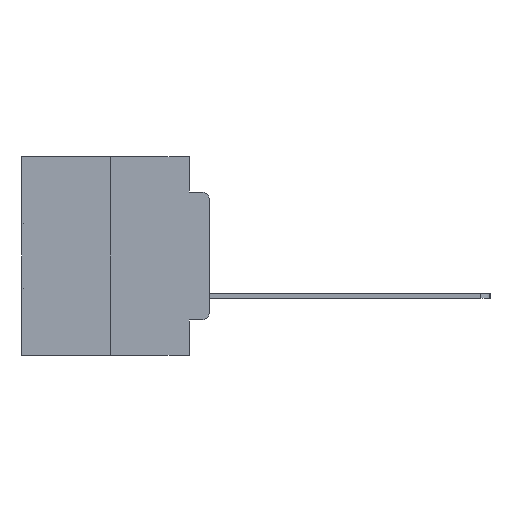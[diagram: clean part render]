
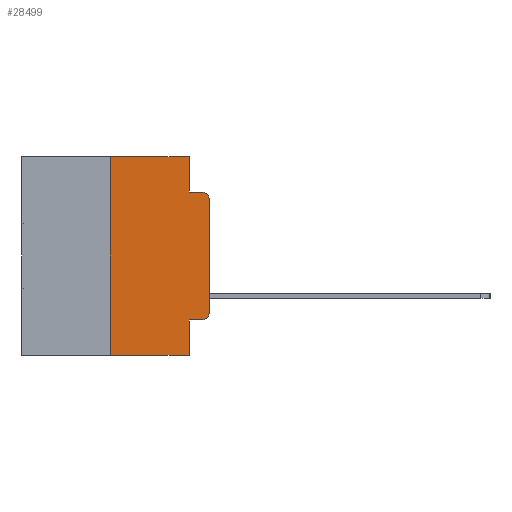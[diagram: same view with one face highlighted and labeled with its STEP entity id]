
A CAD part, left-side view. The second image highlights one B-rep face of the part: STEP entity #28499.
In plain terms, the highlighted planar face has unit normal (-1, 0, 0).
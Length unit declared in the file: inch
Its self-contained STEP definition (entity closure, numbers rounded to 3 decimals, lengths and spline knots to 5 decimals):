
#213 = CARTESIAN_POINT ( 'NONE',  ( 0., 0.02, -0.1085 ) ) ;
#919 = ORIENTED_EDGE ( 'NONE', *, *, #4600, .F. ) ;
#1004 = EDGE_LOOP ( 'NONE', ( #18325, #6069, #16161, #3114, #25255, #919, #17935, #4923, #3471, #26992 ) ) ;
#1137 = EDGE_CURVE ( 'NONE', #25202, #6873, #22551, .T. ) ;
#1201 = VERTEX_POINT ( 'NONE', #24159 ) ;
#1236 = CARTESIAN_POINT ( 'NONE',  ( 0., 0.051, 0. ) ) ;
#1256 = AXIS2_PLACEMENT_3D ( 'NONE', #26044, #12559, #28263 ) ;
#1947 = EDGE_CURVE ( 'NONE', #4671, #1201, #26779, .T. ) ;
#2197 = CARTESIAN_POINT ( 'NONE',  ( 0., 0.473, -0.5 ) ) ;
#2597 = DIRECTION ( 'NONE',  ( 0., 0., -1. ) ) ;
#3114 = ORIENTED_EDGE ( 'NONE', *, *, #23697, .F. ) ;
#3237 = VERTEX_POINT ( 'NONE', #17011 ) ;
#3417 = DIRECTION ( 'NONE',  ( 0., -1., 0. ) ) ;
#3471 = ORIENTED_EDGE ( 'NONE', *, *, #26192, .T. ) ;
#3637 = CARTESIAN_POINT ( 'NONE',  ( 0., 0.051, 0. ) ) ;
#4600 = EDGE_CURVE ( 'NONE', #4671, #25202, #4941, .T. ) ;
#4671 = VERTEX_POINT ( 'NONE', #14330 ) ;
#4902 = CARTESIAN_POINT ( 'NONE',  ( 0., 0.051, -0.4115 ) ) ;
#4923 = ORIENTED_EDGE ( 'NONE', *, *, #5903, .F. ) ;
#4941 = LINE ( 'NONE', #10071, #10447 ) ;
#5130 = CARTESIAN_POINT ( 'NONE',  ( 0., 0.02, -0.4115 ) ) ;
#5691 = AXIS2_PLACEMENT_3D ( 'NONE', #213, #16438, #2597 ) ;
#5903 = EDGE_CURVE ( 'NONE', #13832, #1201, #22442, .T. ) ;
#6069 = ORIENTED_EDGE ( 'NONE', *, *, #29288, .T. ) ;
#6700 = DIRECTION ( 'NONE',  ( 0., 0., 1. ) ) ;
#6873 = VERTEX_POINT ( 'NONE', #3637 ) ;
#7028 = DIRECTION ( 'NONE',  ( 0., 0., -1. ) ) ;
#8142 = DIRECTION ( 'NONE',  ( 0., 0., -1. ) ) ;
#9279 = DIRECTION ( 'NONE',  ( 0., -1., 0. ) ) ;
#9761 = VECTOR ( 'NONE', #13877, 39.37008 ) ;
#10071 = CARTESIAN_POINT ( 'NONE',  ( 0., 0.25, 0. ) ) ;
#10271 = CARTESIAN_POINT ( 'NONE',  ( 0., 0.25, 0. ) ) ;
#10447 = VECTOR ( 'NONE', #6700, 39.37008 ) ;
#10914 = CARTESIAN_POINT ( 'NONE',  ( 0., 0.051, -0.4115 ) ) ;
#11629 = CARTESIAN_POINT ( 'NONE',  ( 0., 0.473, 0. ) ) ;
#11756 = CARTESIAN_POINT ( 'NONE',  ( 0., 0.051, 0. ) ) ;
#12559 = DIRECTION ( 'NONE',  ( -1., 0., 0. ) ) ;
#13060 = FACE_OUTER_BOUND ( 'NONE', #1004, .T. ) ;
#13832 = VERTEX_POINT ( 'NONE', #10914 ) ;
#13877 = DIRECTION ( 'NONE',  ( 0., 0., 1. ) ) ;
#14184 = VERTEX_POINT ( 'NONE', #19039 ) ;
#14330 = CARTESIAN_POINT ( 'NONE',  ( 0., 0.25, -0.5 ) ) ;
#14562 = VERTEX_POINT ( 'NONE', #24772 ) ;
#14836 = CARTESIAN_POINT ( 'NONE',  ( 0., 0.02, -0.0885 ) ) ;
#15877 = LINE ( 'NONE', #27285, #9761 ) ;
#16003 = EDGE_CURVE ( 'NONE', #25725, #3237, #29301, .T. ) ;
#16050 = LINE ( 'NONE', #19537, #21341 ) ;
#16052 = EDGE_CURVE ( 'NONE', #14184, #16690, #16050, .T. ) ;
#16161 = ORIENTED_EDGE ( 'NONE', *, *, #16052, .F. ) ;
#16219 = DIRECTION ( 'NONE',  ( 0., 0., -1. ) ) ;
#16438 = DIRECTION ( 'NONE',  ( -1., 0., 0. ) ) ;
#16690 = VERTEX_POINT ( 'NONE', #14836 ) ;
#17011 = CARTESIAN_POINT ( 'NONE',  ( 0., 0., -0.3915 ) ) ;
#17935 = ORIENTED_EDGE ( 'NONE', *, *, #1947, .T. ) ;
#18325 = ORIENTED_EDGE ( 'NONE', *, *, #27883, .T. ) ;
#18706 = DIRECTION ( 'NONE',  ( 0., -1., 0. ) ) ;
#19039 = CARTESIAN_POINT ( 'NONE',  ( 0., 0.051, -0.0885 ) ) ;
#19145 = VECTOR ( 'NONE', #8142, 39.37008 ) ;
#19537 = CARTESIAN_POINT ( 'NONE',  ( 0., 0.051, -0.0885 ) ) ;
#19883 = LINE ( 'NONE', #1236, #19145 ) ;
#20569 = DIRECTION ( 'NONE',  ( 0., -1., 0. ) ) ;
#20880 = VECTOR ( 'NONE', #20569, 39.37008 ) ;
#21341 = VECTOR ( 'NONE', #3417, 39.37008 ) ;
#21862 = VECTOR ( 'NONE', #9279, 39.37008 ) ;
#22442 = LINE ( 'NONE', #11756, #27602 ) ;
#22551 = LINE ( 'NONE', #22916, #21862 ) ;
#22916 = CARTESIAN_POINT ( 'NONE',  ( 0., 0.473, 0. ) ) ;
#23376 = LINE ( 'NONE', #4902, #29241 ) ;
#23697 = EDGE_CURVE ( 'NONE', #6873, #14184, #19883, .T. ) ;
#24159 = CARTESIAN_POINT ( 'NONE',  ( 0., 0.051, -0.5 ) ) ;
#24772 = CARTESIAN_POINT ( 'NONE',  ( 0., 0., -0.1085 ) ) ;
#25202 = VERTEX_POINT ( 'NONE', #10271 ) ;
#25255 = ORIENTED_EDGE ( 'NONE', *, *, #1137, .F. ) ;
#25725 = VERTEX_POINT ( 'NONE', #5130 ) ;
#26044 = CARTESIAN_POINT ( 'NONE',  ( 0., 0.02, -0.3915 ) ) ;
#26192 = EDGE_CURVE ( 'NONE', #13832, #25725, #23376, .T. ) ;
#26779 = LINE ( 'NONE', #2197, #20880 ) ;
#26992 = ORIENTED_EDGE ( 'NONE', *, *, #16003, .T. ) ;
#27060 = CIRCLE ( 'NONE', #5691, 0.02 ) ;
#27285 = CARTESIAN_POINT ( 'NONE',  ( 0., 0., 0. ) ) ;
#27347 = PLANE ( 'NONE',  #27724 ) ;
#27602 = VECTOR ( 'NONE', #7028, 39.37008 ) ;
#27724 = AXIS2_PLACEMENT_3D ( 'NONE', #11629, #28920, #16219 ) ;
#27883 = EDGE_CURVE ( 'NONE', #3237, #14562, #15877, .T. ) ;
#28263 = DIRECTION ( 'NONE',  ( 0., 0., -1. ) ) ;
#28499 = ADVANCED_FACE ( 'NONE', ( #13060 ), #27347, .F. ) ;
#28920 = DIRECTION ( 'NONE',  ( 1., 0., 0. ) ) ;
#29241 = VECTOR ( 'NONE', #18706, 39.37008 ) ;
#29288 = EDGE_CURVE ( 'NONE', #14562, #16690, #27060, .T. ) ;
#29301 = CIRCLE ( 'NONE', #1256, 0.02 ) ;
